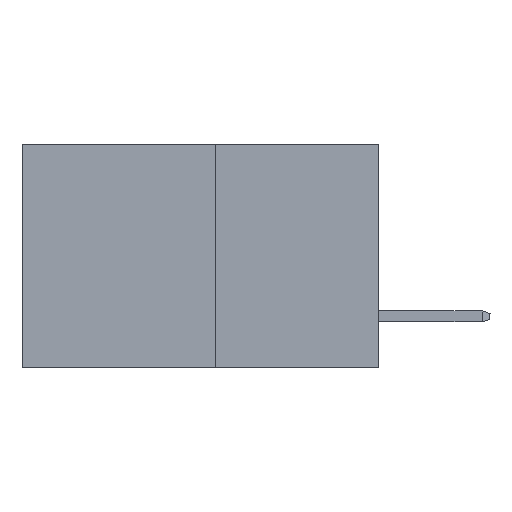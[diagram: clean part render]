
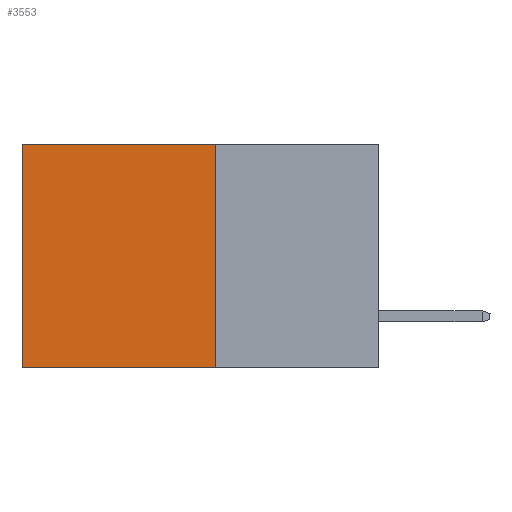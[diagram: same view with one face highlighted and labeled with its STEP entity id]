
A CAD part, left-side view. The second image highlights one B-rep face of the part: STEP entity #3553.
In plain terms, the highlighted planar face has unit normal (-1, 0, 0).
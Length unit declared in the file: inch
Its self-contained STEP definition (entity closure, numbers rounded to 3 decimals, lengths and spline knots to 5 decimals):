
#486 = LINE ( 'NONE', #819, #7537 ) ;
#819 = CARTESIAN_POINT ( 'NONE',  ( 0.277, 0.27, -0.37 ) ) ;
#1155 = VERTEX_POINT ( 'NONE', #7220 ) ;
#1453 = ORIENTED_EDGE ( 'NONE', *, *, #6430, .F. ) ;
#1620 = DIRECTION ( 'NONE',  ( 1., 0., 0. ) ) ;
#1633 = LINE ( 'NONE', #4788, #2259 ) ;
#1701 = VERTEX_POINT ( 'NONE', #7345 ) ;
#2259 = VECTOR ( 'NONE', #11104, 39.37008 ) ;
#2411 = AXIS2_PLACEMENT_3D ( 'NONE', #2946, #1620, #2443 ) ;
#2443 = DIRECTION ( 'NONE',  ( 0., 0., -1. ) ) ;
#2469 = EDGE_LOOP ( 'NONE', ( #8915, #1453, #10998, #8936 ) ) ;
#2486 = EDGE_CURVE ( 'NONE', #1155, #7934, #3176, .T. ) ;
#2946 = CARTESIAN_POINT ( 'NONE',  ( 0.277, 0.27, -0.37 ) ) ;
#2971 = EDGE_CURVE ( 'NONE', #7934, #10757, #1633, .T. ) ;
#3176 = LINE ( 'NONE', #4627, #5951 ) ;
#3404 = CARTESIAN_POINT ( 'NONE',  ( 0.277, 0.27, -0.37 ) ) ;
#3553 = ADVANCED_FACE ( 'NONE', ( #3742 ), #10881, .F. ) ;
#3742 = FACE_OUTER_BOUND ( 'NONE', #2469, .T. ) ;
#4055 = CARTESIAN_POINT ( 'NONE',  ( 0.277, 0.59, -0.37 ) ) ;
#4627 = CARTESIAN_POINT ( 'NONE',  ( 0.277, 0.27, 0. ) ) ;
#4788 = CARTESIAN_POINT ( 'NONE',  ( 0.277, 0.59, -0.37 ) ) ;
#5636 = DIRECTION ( 'NONE',  ( 0., 1., 0. ) ) ;
#5951 = VECTOR ( 'NONE', #5636, 39.37008 ) ;
#6424 = DIRECTION ( 'NONE',  ( 0., 1., 0. ) ) ;
#6430 = EDGE_CURVE ( 'NONE', #1701, #10757, #486, .T. ) ;
#6995 = DIRECTION ( 'NONE',  ( 0., 0., -1. ) ) ;
#7220 = CARTESIAN_POINT ( 'NONE',  ( 0.277, 0.27, 0. ) ) ;
#7345 = CARTESIAN_POINT ( 'NONE',  ( 0.277, 0.27, -0.37 ) ) ;
#7537 = VECTOR ( 'NONE', #6424, 39.37008 ) ;
#7681 = EDGE_CURVE ( 'NONE', #1155, #1701, #10273, .T. ) ;
#7934 = VERTEX_POINT ( 'NONE', #8329 ) ;
#8066 = VECTOR ( 'NONE', #6995, 39.37008 ) ;
#8329 = CARTESIAN_POINT ( 'NONE',  ( 0.277, 0.59, 0. ) ) ;
#8915 = ORIENTED_EDGE ( 'NONE', *, *, #2971, .T. ) ;
#8936 = ORIENTED_EDGE ( 'NONE', *, *, #2486, .T. ) ;
#10273 = LINE ( 'NONE', #3404, #8066 ) ;
#10757 = VERTEX_POINT ( 'NONE', #4055 ) ;
#10881 = PLANE ( 'NONE',  #2411 ) ;
#10998 = ORIENTED_EDGE ( 'NONE', *, *, #7681, .F. ) ;
#11104 = DIRECTION ( 'NONE',  ( 0., 0., -1. ) ) ;
